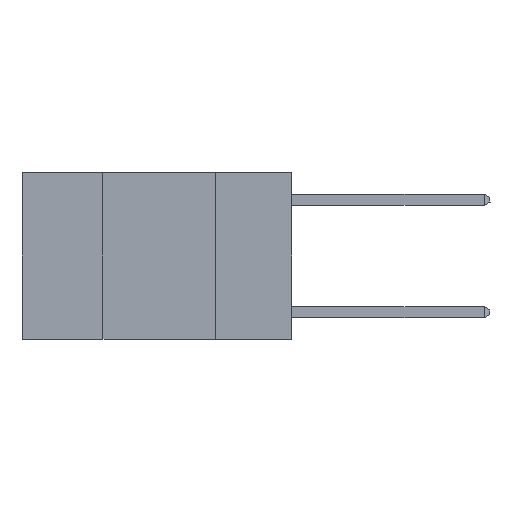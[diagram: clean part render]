
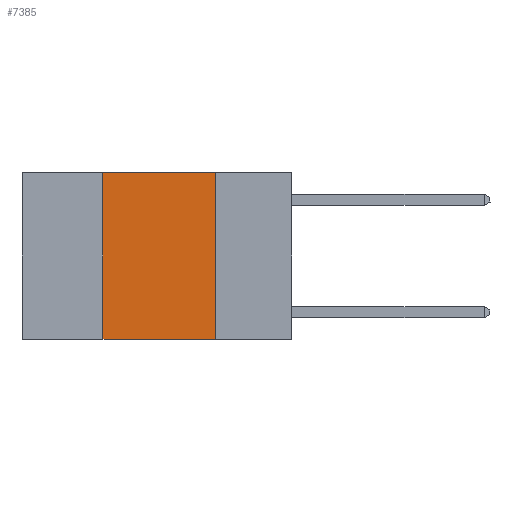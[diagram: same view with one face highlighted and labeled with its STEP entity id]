
A CAD part, left-side view. The second image highlights one B-rep face of the part: STEP entity #7385.
In plain terms, the highlighted planar face has unit normal (-1, 0, 0).
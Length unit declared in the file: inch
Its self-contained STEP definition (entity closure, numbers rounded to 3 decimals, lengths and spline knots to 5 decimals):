
#277 = CARTESIAN_POINT ( 'NONE',  ( 0., 0.17, 0. ) ) ;
#328 = VERTEX_POINT ( 'NONE', #15716 ) ;
#735 = CARTESIAN_POINT ( 'NONE',  ( 0., 0.6, 0. ) ) ;
#740 = EDGE_LOOP ( 'NONE', ( #6566, #6963, #8939, #8774 ) ) ;
#975 = CARTESIAN_POINT ( 'NONE',  ( 0., 0.17, -0.37 ) ) ;
#1493 = EDGE_CURVE ( 'NONE', #15017, #4446, #5674, .T. ) ;
#2166 = LINE ( 'NONE', #6388, #11197 ) ;
#2250 = EDGE_CURVE ( 'NONE', #15017, #328, #2166, .T. ) ;
#2912 = VECTOR ( 'NONE', #7730, 39.37008 ) ;
#3009 = DIRECTION ( 'NONE',  ( 0., 0., 1. ) ) ;
#3081 = LINE ( 'NONE', #277, #2912 ) ;
#3433 = VERTEX_POINT ( 'NONE', #11215 ) ;
#3860 = FACE_OUTER_BOUND ( 'NONE', #740, .T. ) ;
#4446 = VERTEX_POINT ( 'NONE', #975 ) ;
#4474 = DIRECTION ( 'NONE',  ( 0., 0., -1. ) ) ;
#4677 = LINE ( 'NONE', #5429, #10814 ) ;
#5429 = CARTESIAN_POINT ( 'NONE',  ( 0., 0.6, 0. ) ) ;
#5674 = LINE ( 'NONE', #14236, #12901 ) ;
#5999 = EDGE_CURVE ( 'NONE', #328, #3433, #4677, .T. ) ;
#6388 = CARTESIAN_POINT ( 'NONE',  ( 0., 0.42, 0. ) ) ;
#6566 = ORIENTED_EDGE ( 'NONE', *, *, #10813, .F. ) ;
#6859 = CARTESIAN_POINT ( 'NONE',  ( 0., 0.42, -0.37 ) ) ;
#6963 = ORIENTED_EDGE ( 'NONE', *, *, #5999, .F. ) ;
#7385 = ADVANCED_FACE ( 'NONE', ( #3860 ), #10598, .F. ) ;
#7730 = DIRECTION ( 'NONE',  ( 0., 0., -1. ) ) ;
#8774 = ORIENTED_EDGE ( 'NONE', *, *, #1493, .T. ) ;
#8939 = ORIENTED_EDGE ( 'NONE', *, *, #2250, .F. ) ;
#10598 = PLANE ( 'NONE',  #11656 ) ;
#10813 = EDGE_CURVE ( 'NONE', #3433, #4446, #3081, .T. ) ;
#10814 = VECTOR ( 'NONE', #12719, 39.37008 ) ;
#11197 = VECTOR ( 'NONE', #3009, 39.37008 ) ;
#11215 = CARTESIAN_POINT ( 'NONE',  ( 0., 0.17, 0. ) ) ;
#11656 = AXIS2_PLACEMENT_3D ( 'NONE', #735, #11794, #4474 ) ;
#11794 = DIRECTION ( 'NONE',  ( 1., 0., 0. ) ) ;
#12719 = DIRECTION ( 'NONE',  ( 0., -1., 0. ) ) ;
#12901 = VECTOR ( 'NONE', #15373, 39.37008 ) ;
#14236 = CARTESIAN_POINT ( 'NONE',  ( 0., 0.6, -0.37 ) ) ;
#15017 = VERTEX_POINT ( 'NONE', #6859 ) ;
#15373 = DIRECTION ( 'NONE',  ( 0., -1., 0. ) ) ;
#15716 = CARTESIAN_POINT ( 'NONE',  ( 0., 0.42, 0. ) ) ;
